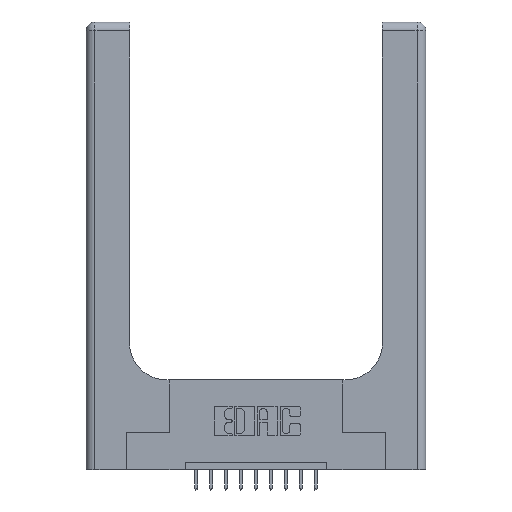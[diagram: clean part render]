
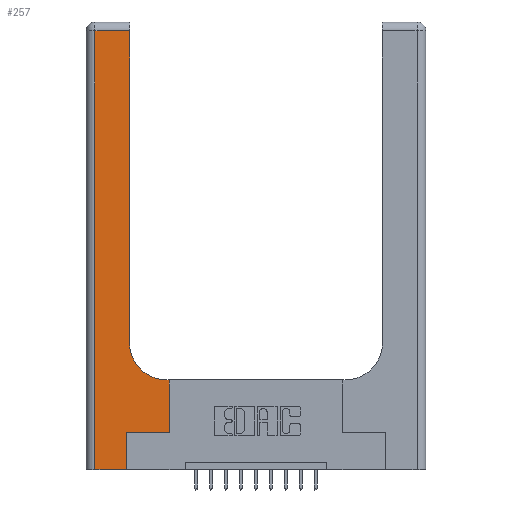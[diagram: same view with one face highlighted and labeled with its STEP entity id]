
A CAD part, top view. The second image highlights one B-rep face of the part: STEP entity #257.
In plain terms, the highlighted planar face has unit normal (0, 0, 1).
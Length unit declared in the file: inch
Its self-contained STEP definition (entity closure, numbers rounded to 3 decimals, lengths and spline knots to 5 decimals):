
#82 = CARTESIAN_POINT ( 'NONE',  ( 0.269, 0., 0.37 ) ) ;
#257 = ADVANCED_FACE ( 'NONE', ( #7293 ), #4630, .F. ) ;
#270 = EDGE_CURVE ( 'NONE', #15453, #5385, #10566, .T. ) ;
#299 = CARTESIAN_POINT ( 'NONE',  ( 0.5415, 0.6, 0.37 ) ) ;
#574 = ORIENTED_EDGE ( 'NONE', *, *, #270, .T. ) ;
#651 = CARTESIAN_POINT ( 'NONE',  ( 0.5585, 0.6, 0.37 ) ) ;
#951 = DIRECTION ( 'NONE',  ( 0., 0., -1. ) ) ;
#952 = VERTEX_POINT ( 'NONE', #3096 ) ;
#961 = DIRECTION ( 'NONE',  ( -1., 0., 0. ) ) ;
#1005 = VECTOR ( 'NONE', #8964, 39.37008 ) ;
#1392 = EDGE_CURVE ( 'NONE', #14123, #14888, #15673, .T. ) ;
#1492 = EDGE_CURVE ( 'NONE', #952, #7308, #6457, .T. ) ;
#2213 = CARTESIAN_POINT ( 'NONE',  ( 0.2915, 0.6, 0.37 ) ) ;
#2648 = DIRECTION ( 'NONE',  ( 1., 0., 0. ) ) ;
#3096 = CARTESIAN_POINT ( 'NONE',  ( 0.269, 0.25, 0.37 ) ) ;
#3117 = EDGE_CURVE ( 'NONE', #15757, #952, #10250, .T. ) ;
#3151 = LINE ( 'NONE', #4569, #3418 ) ;
#3418 = VECTOR ( 'NONE', #12072, 39.37008 ) ;
#3466 = CARTESIAN_POINT ( 'NONE',  ( 0.5415, 0.85, 0.37 ) ) ;
#3586 = CARTESIAN_POINT ( 'NONE',  ( 0.5585, 0.25, 0.37 ) ) ;
#3806 = EDGE_CURVE ( 'NONE', #14888, #12024, #13110, .T. ) ;
#3898 = LINE ( 'NONE', #14071, #10941 ) ;
#3964 = LINE ( 'NONE', #10134, #5232 ) ;
#4108 = CARTESIAN_POINT ( 'NONE',  ( 0.06, 3., 0.37 ) ) ;
#4569 = CARTESIAN_POINT ( 'NONE',  ( 0.5585, 0.25, 0.37 ) ) ;
#4630 = PLANE ( 'NONE',  #6305 ) ;
#4951 = EDGE_CURVE ( 'NONE', #6058, #15453, #13640, .T. ) ;
#5232 = VECTOR ( 'NONE', #7718, 39.37008 ) ;
#5237 = ORIENTED_EDGE ( 'NONE', *, *, #1492, .T. ) ;
#5385 = VERTEX_POINT ( 'NONE', #15284 ) ;
#5671 = EDGE_LOOP ( 'NONE', ( #10609, #13056, #13695, #11688, #12074, #5237, #16358, #10835, #574 ) ) ;
#5895 = EDGE_CURVE ( 'NONE', #12024, #15757, #3898, .T. ) ;
#6040 = DIRECTION ( 'NONE',  ( 1., 0., 0. ) ) ;
#6058 = VERTEX_POINT ( 'NONE', #651 ) ;
#6293 = CARTESIAN_POINT ( 'NONE',  ( 0.06, 0., 0.37 ) ) ;
#6305 = AXIS2_PLACEMENT_3D ( 'NONE', #14889, #13470, #9572 ) ;
#6457 = LINE ( 'NONE', #12536, #1005 ) ;
#6919 = VECTOR ( 'NONE', #11677, 39.37008 ) ;
#7293 = FACE_OUTER_BOUND ( 'NONE', #5671, .T. ) ;
#7308 = VERTEX_POINT ( 'NONE', #3586 ) ;
#7623 = AXIS2_PLACEMENT_3D ( 'NONE', #3466, #951, #6040 ) ;
#7718 = DIRECTION ( 'NONE',  ( 0., 1., 0. ) ) ;
#7940 = CARTESIAN_POINT ( 'NONE',  ( 0.06, 2.94, 0.37 ) ) ;
#8959 = EDGE_CURVE ( 'NONE', #7308, #6058, #3151, .T. ) ;
#8964 = DIRECTION ( 'NONE',  ( 1., 0., 0. ) ) ;
#9204 = DIRECTION ( 'NONE',  ( 0., -1., 0. ) ) ;
#9572 = DIRECTION ( 'NONE',  ( -1., 0., 0. ) ) ;
#10073 = VECTOR ( 'NONE', #9204, 39.37008 ) ;
#10134 = CARTESIAN_POINT ( 'NONE',  ( 0.2915, 3., 0.37 ) ) ;
#10250 = LINE ( 'NONE', #82, #6919 ) ;
#10566 = CIRCLE ( 'NONE', #7623, 0.25 ) ;
#10609 = ORIENTED_EDGE ( 'NONE', *, *, #13131, .T. ) ;
#10835 = ORIENTED_EDGE ( 'NONE', *, *, #4951, .T. ) ;
#10941 = VECTOR ( 'NONE', #2648, 39.37008 ) ;
#11434 = VECTOR ( 'NONE', #961, 39.37008 ) ;
#11677 = DIRECTION ( 'NONE',  ( 0., 1., 0. ) ) ;
#11688 = ORIENTED_EDGE ( 'NONE', *, *, #5895, .T. ) ;
#12007 = DIRECTION ( 'NONE',  ( -1., 0., 0. ) ) ;
#12024 = VERTEX_POINT ( 'NONE', #6293 ) ;
#12072 = DIRECTION ( 'NONE',  ( 0., 1., 0. ) ) ;
#12074 = ORIENTED_EDGE ( 'NONE', *, *, #3117, .T. ) ;
#12536 = CARTESIAN_POINT ( 'NONE',  ( 0.269, 0.25, 0.37 ) ) ;
#13056 = ORIENTED_EDGE ( 'NONE', *, *, #1392, .T. ) ;
#13110 = LINE ( 'NONE', #4108, #10073 ) ;
#13131 = EDGE_CURVE ( 'NONE', #5385, #14123, #3964, .T. ) ;
#13470 = DIRECTION ( 'NONE',  ( 0., 0., -1. ) ) ;
#13527 = VECTOR ( 'NONE', #12007, 39.37008 ) ;
#13619 = CARTESIAN_POINT ( 'NONE',  ( 0.269, 0., 0.37 ) ) ;
#13640 = LINE ( 'NONE', #2213, #11434 ) ;
#13695 = ORIENTED_EDGE ( 'NONE', *, *, #3806, .T. ) ;
#14071 = CARTESIAN_POINT ( 'NONE',  ( 0., 0., 0.37 ) ) ;
#14123 = VERTEX_POINT ( 'NONE', #16085 ) ;
#14888 = VERTEX_POINT ( 'NONE', #7940 ) ;
#14889 = CARTESIAN_POINT ( 'NONE',  ( 0., 3., 0.37 ) ) ;
#15284 = CARTESIAN_POINT ( 'NONE',  ( 0.2915, 0.85, 0.37 ) ) ;
#15453 = VERTEX_POINT ( 'NONE', #299 ) ;
#15673 = LINE ( 'NONE', #15921, #13527 ) ;
#15757 = VERTEX_POINT ( 'NONE', #13619 ) ;
#15921 = CARTESIAN_POINT ( 'NONE',  ( 0., 2.94, 0.37 ) ) ;
#16085 = CARTESIAN_POINT ( 'NONE',  ( 0.2915, 2.94, 0.37 ) ) ;
#16358 = ORIENTED_EDGE ( 'NONE', *, *, #8959, .T. ) ;
